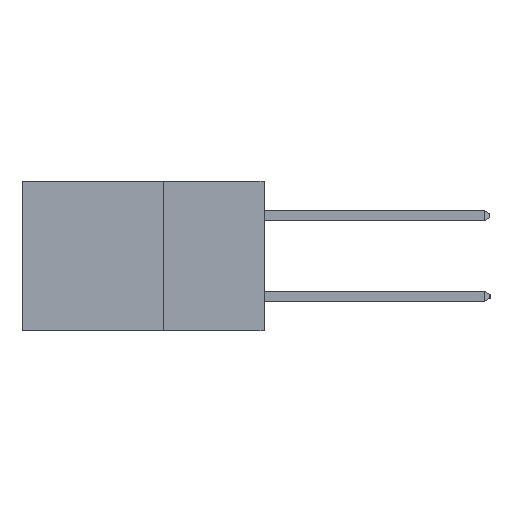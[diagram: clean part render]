
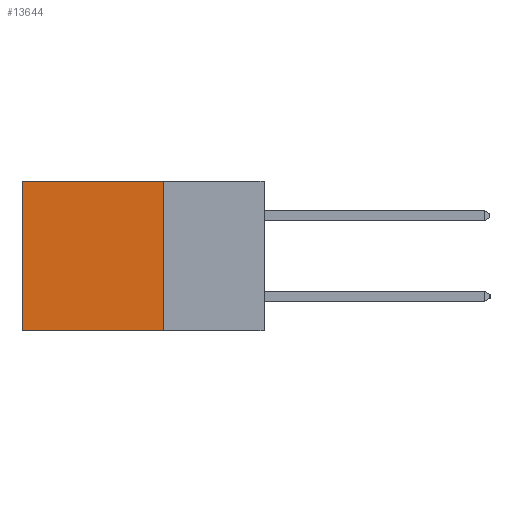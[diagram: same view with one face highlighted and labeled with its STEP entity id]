
A CAD part, left-side view. The second image highlights one B-rep face of the part: STEP entity #13644.
In plain terms, the highlighted planar face has unit normal (-1, 0, 0).
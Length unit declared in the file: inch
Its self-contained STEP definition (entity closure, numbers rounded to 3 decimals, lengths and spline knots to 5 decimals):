
#13 = EDGE_CURVE ( 'NONE', #17713, #5807, #21271, .T. ) ;
#218 = EDGE_CURVE ( 'NONE', #13169, #17642, #9412, .T. ) ;
#1486 = CARTESIAN_POINT ( 'NONE',  ( 0.2615, 0.6, -0.37 ) ) ;
#2168 = AXIS2_PLACEMENT_3D ( 'NONE', #13174, #2638, #14928 ) ;
#2638 = DIRECTION ( 'NONE',  ( 1., 0., 0. ) ) ;
#5747 = DIRECTION ( 'NONE',  ( 0., 1., 0. ) ) ;
#5807 = VERTEX_POINT ( 'NONE', #1486 ) ;
#5830 = EDGE_CURVE ( 'NONE', #17642, #5807, #20343, .T. ) ;
#6123 = CARTESIAN_POINT ( 'NONE',  ( 0.2615, 0.25, 0. ) ) ;
#7794 = ORIENTED_EDGE ( 'NONE', *, *, #218, .T. ) ;
#7924 = PLANE ( 'NONE',  #2168 ) ;
#8518 = ORIENTED_EDGE ( 'NONE', *, *, #5830, .T. ) ;
#8536 = CARTESIAN_POINT ( 'NONE',  ( 0.2615, 0.25, -0.37 ) ) ;
#9320 = EDGE_CURVE ( 'NONE', #13169, #17713, #13715, .T. ) ;
#9412 = LINE ( 'NONE', #6123, #18590 ) ;
#9662 = CARTESIAN_POINT ( 'NONE',  ( 0.2615, 0.25, -0.37 ) ) ;
#11170 = VECTOR ( 'NONE', #15642, 39.37008 ) ;
#11428 = ORIENTED_EDGE ( 'NONE', *, *, #13, .F. ) ;
#11878 = EDGE_LOOP ( 'NONE', ( #8518, #11428, #20755, #7794 ) ) ;
#13169 = VERTEX_POINT ( 'NONE', #20082 ) ;
#13174 = CARTESIAN_POINT ( 'NONE',  ( 0.2615, 0.25, -0.37 ) ) ;
#13644 = ADVANCED_FACE ( 'NONE', ( #14136 ), #7924, .F. ) ;
#13715 = LINE ( 'NONE', #9662, #14247 ) ;
#13904 = CARTESIAN_POINT ( 'NONE',  ( 0.2615, 0.6, -0.37 ) ) ;
#14136 = FACE_OUTER_BOUND ( 'NONE', #11878, .T. ) ;
#14247 = VECTOR ( 'NONE', #21711, 39.37008 ) ;
#14928 = DIRECTION ( 'NONE',  ( 0., 0., -1. ) ) ;
#15642 = DIRECTION ( 'NONE',  ( 0., 0., -1. ) ) ;
#16492 = CARTESIAN_POINT ( 'NONE',  ( 0.2615, 0.25, -0.37 ) ) ;
#16753 = VECTOR ( 'NONE', #18137, 39.37008 ) ;
#17642 = VERTEX_POINT ( 'NONE', #22098 ) ;
#17713 = VERTEX_POINT ( 'NONE', #8536 ) ;
#18137 = DIRECTION ( 'NONE',  ( 0., 1., 0. ) ) ;
#18590 = VECTOR ( 'NONE', #5747, 39.37008 ) ;
#20082 = CARTESIAN_POINT ( 'NONE',  ( 0.2615, 0.25, 0. ) ) ;
#20343 = LINE ( 'NONE', #13904, #11170 ) ;
#20755 = ORIENTED_EDGE ( 'NONE', *, *, #9320, .F. ) ;
#21271 = LINE ( 'NONE', #16492, #16753 ) ;
#21711 = DIRECTION ( 'NONE',  ( 0., 0., -1. ) ) ;
#22098 = CARTESIAN_POINT ( 'NONE',  ( 0.2615, 0.6, 0. ) ) ;
